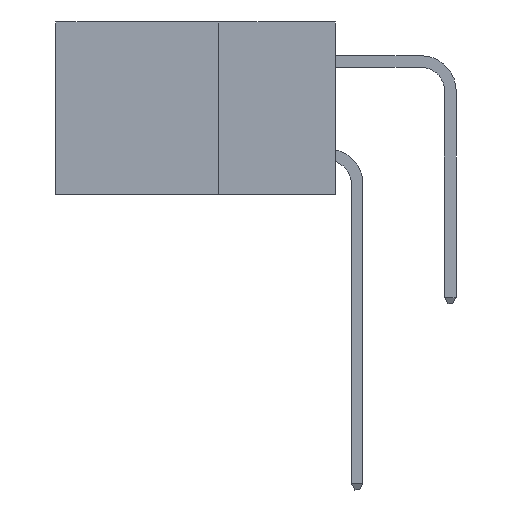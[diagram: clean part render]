
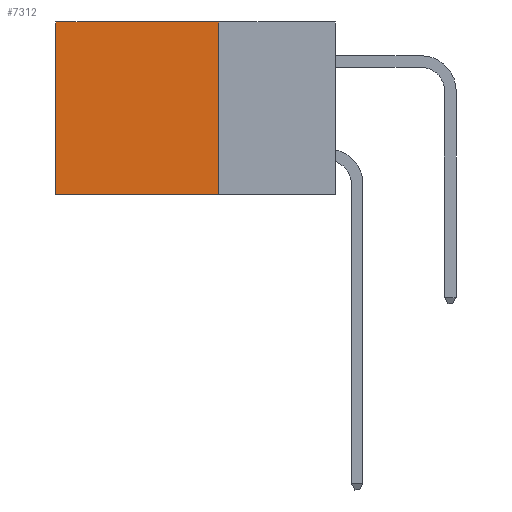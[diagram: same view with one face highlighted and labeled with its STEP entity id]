
A CAD part, left-side view. The second image highlights one B-rep face of the part: STEP entity #7312.
In plain terms, the highlighted planar face has unit normal (-1, 0, 0).
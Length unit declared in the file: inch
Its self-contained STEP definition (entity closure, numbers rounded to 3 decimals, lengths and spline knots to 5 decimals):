
#1365 = LINE ( 'NONE', #7760, #15434 ) ;
#1776 = VECTOR ( 'NONE', #4058, 39.37008 ) ;
#2652 = LINE ( 'NONE', #16189, #1776 ) ;
#2776 = ORIENTED_EDGE ( 'NONE', *, *, #12723, .F. ) ;
#3031 = VERTEX_POINT ( 'NONE', #15956 ) ;
#4058 = DIRECTION ( 'NONE',  ( 0., 1., 0. ) ) ;
#4368 = VERTEX_POINT ( 'NONE', #13231 ) ;
#4983 = VECTOR ( 'NONE', #7244, 39.37008 ) ;
#5290 = VERTEX_POINT ( 'NONE', #14047 ) ;
#5429 = ORIENTED_EDGE ( 'NONE', *, *, #9216, .T. ) ;
#5503 = DIRECTION ( 'NONE',  ( 0., 0., -1. ) ) ;
#6041 = LINE ( 'NONE', #9562, #13640 ) ;
#6321 = EDGE_CURVE ( 'NONE', #16579, #5290, #2652, .T. ) ;
#7244 = DIRECTION ( 'NONE',  ( 0., 0., -1. ) ) ;
#7312 = ADVANCED_FACE ( 'NONE', ( #14979 ), #8063, .F. ) ;
#7760 = CARTESIAN_POINT ( 'NONE',  ( 0.2875, 0.25, 0. ) ) ;
#8063 = PLANE ( 'NONE',  #10176 ) ;
#8851 = ORIENTED_EDGE ( 'NONE', *, *, #9654, .T. ) ;
#8987 = LINE ( 'NONE', #13995, #4983 ) ;
#9216 = EDGE_CURVE ( 'NONE', #3031, #5290, #6041, .T. ) ;
#9434 = DIRECTION ( 'NONE',  ( 0., 0., -1. ) ) ;
#9562 = CARTESIAN_POINT ( 'NONE',  ( 0.2875, 0.6, 0. ) ) ;
#9632 = ORIENTED_EDGE ( 'NONE', *, *, #6321, .F. ) ;
#9654 = EDGE_CURVE ( 'NONE', #4368, #3031, #1365, .T. ) ;
#10176 = AXIS2_PLACEMENT_3D ( 'NONE', #14808, #17485, #9434 ) ;
#12723 = EDGE_CURVE ( 'NONE', #4368, #16579, #8987, .T. ) ;
#13231 = CARTESIAN_POINT ( 'NONE',  ( 0.2875, 0.25, 0. ) ) ;
#13640 = VECTOR ( 'NONE', #5503, 39.37008 ) ;
#13995 = CARTESIAN_POINT ( 'NONE',  ( 0.2875, 0.25, 0. ) ) ;
#14047 = CARTESIAN_POINT ( 'NONE',  ( 0.2875, 0.6, -0.37 ) ) ;
#14808 = CARTESIAN_POINT ( 'NONE',  ( 0.2875, 0.25, 0. ) ) ;
#14979 = FACE_OUTER_BOUND ( 'NONE', #15380, .T. ) ;
#15380 = EDGE_LOOP ( 'NONE', ( #5429, #9632, #2776, #8851 ) ) ;
#15434 = VECTOR ( 'NONE', #17179, 39.37008 ) ;
#15956 = CARTESIAN_POINT ( 'NONE',  ( 0.2875, 0.6, 0. ) ) ;
#16189 = CARTESIAN_POINT ( 'NONE',  ( 0.2875, 0.25, -0.37 ) ) ;
#16579 = VERTEX_POINT ( 'NONE', #17173 ) ;
#17173 = CARTESIAN_POINT ( 'NONE',  ( 0.2875, 0.25, -0.37 ) ) ;
#17179 = DIRECTION ( 'NONE',  ( 0., 1., 0. ) ) ;
#17485 = DIRECTION ( 'NONE',  ( 1., 0., 0. ) ) ;
